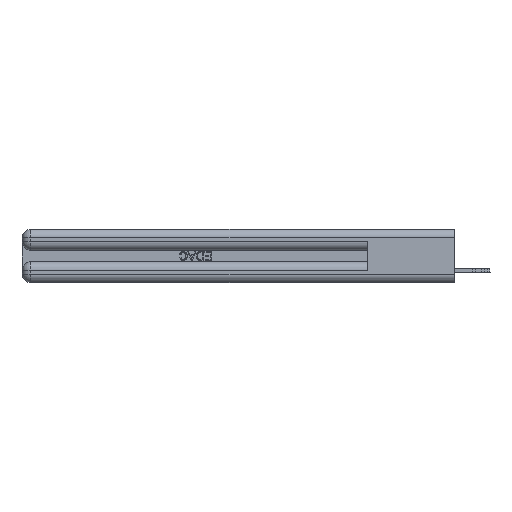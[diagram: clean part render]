
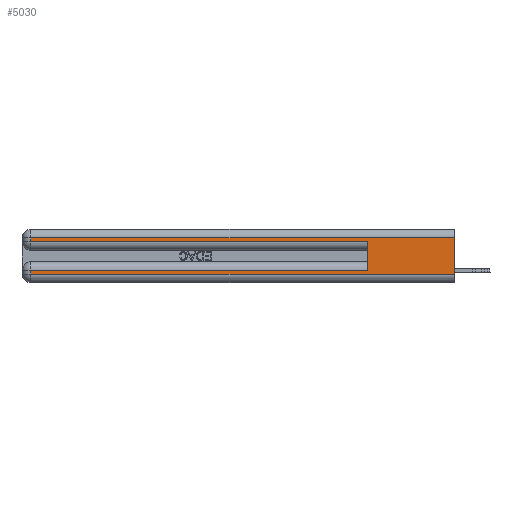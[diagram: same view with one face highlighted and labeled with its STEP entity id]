
A CAD part, left-side view. The second image highlights one B-rep face of the part: STEP entity #5030.
In plain terms, the highlighted planar face has unit normal (-1, 0, 0).
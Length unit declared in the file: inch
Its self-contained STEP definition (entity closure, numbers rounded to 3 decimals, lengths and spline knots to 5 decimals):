
#437 = CARTESIAN_POINT ( 'NONE',  ( 0., 2.94, 0.37 ) ) ;
#770 = DIRECTION ( 'NONE',  ( 1., 0., 0. ) ) ;
#1488 = EDGE_CURVE ( 'NONE', #3719, #33987, #32286, .T. ) ;
#1748 = EDGE_CURVE ( 'NONE', #42653, #26759, #40231, .T. ) ;
#3719 = VERTEX_POINT ( 'NONE', #22581 ) ;
#4705 = VERTEX_POINT ( 'NONE', #6514 ) ;
#5030 = ADVANCED_FACE ( 'NONE', ( #17092 ), #41225, .F. ) ;
#6514 = CARTESIAN_POINT ( 'NONE',  ( 0., 2.94, 0.31 ) ) ;
#7011 = EDGE_CURVE ( 'NONE', #24779, #18152, #34283, .T. ) ;
#9468 = VECTOR ( 'NONE', #13806, 39.37008 ) ;
#11278 = EDGE_CURVE ( 'NONE', #24779, #33987, #25274, .T. ) ;
#11892 = CARTESIAN_POINT ( 'NONE',  ( 0., 2.94, 0.06 ) ) ;
#11975 = DIRECTION ( 'NONE',  ( 0., 1., 0. ) ) ;
#12269 = VERTEX_POINT ( 'NONE', #37901 ) ;
#13163 = ORIENTED_EDGE ( 'NONE', *, *, #1748, .T. ) ;
#13584 = EDGE_CURVE ( 'NONE', #12269, #4705, #14735, .T. ) ;
#13806 = DIRECTION ( 'NONE',  ( 0., -1., 0. ) ) ;
#14131 = CARTESIAN_POINT ( 'NONE',  ( 0., 0.6, 0.285 ) ) ;
#14662 = ORIENTED_EDGE ( 'NONE', *, *, #11278, .F. ) ;
#14735 = LINE ( 'NONE', #26303, #24962 ) ;
#14923 = VECTOR ( 'NONE', #26394, 39.37008 ) ;
#15210 = ORIENTED_EDGE ( 'NONE', *, *, #1488, .T. ) ;
#15259 = AXIS2_PLACEMENT_3D ( 'NONE', #40905, #770, #33738 ) ;
#16176 = ORIENTED_EDGE ( 'NONE', *, *, #39527, .T. ) ;
#16331 = CARTESIAN_POINT ( 'NONE',  ( 0., 0., 0.06 ) ) ;
#17092 = FACE_OUTER_BOUND ( 'NONE', #43045, .T. ) ;
#18152 = VERTEX_POINT ( 'NONE', #25336 ) ;
#18877 = DIRECTION ( 'NONE',  ( 0., 0., 1. ) ) ;
#20898 = VECTOR ( 'NONE', #37984, 39.37008 ) ;
#21423 = DIRECTION ( 'NONE',  ( 0., 0., -1. ) ) ;
#22000 = DIRECTION ( 'NONE',  ( 0., 0., -1. ) ) ;
#22581 = CARTESIAN_POINT ( 'NONE',  ( 0., 2.94, 0.285 ) ) ;
#24779 = VERTEX_POINT ( 'NONE', #44823 ) ;
#24962 = VECTOR ( 'NONE', #11975, 39.37008 ) ;
#25274 = LINE ( 'NONE', #37369, #44666 ) ;
#25336 = CARTESIAN_POINT ( 'NONE',  ( 0., 2.94, 0.085 ) ) ;
#25928 = CARTESIAN_POINT ( 'NONE',  ( 0., 0., 0.085 ) ) ;
#26303 = CARTESIAN_POINT ( 'NONE',  ( 0., 0., 0.31 ) ) ;
#26394 = DIRECTION ( 'NONE',  ( 0., 1., 0. ) ) ;
#26427 = CARTESIAN_POINT ( 'NONE',  ( 0., 2.94, 0.37 ) ) ;
#26759 = VERTEX_POINT ( 'NONE', #33015 ) ;
#29350 = EDGE_CURVE ( 'NONE', #12269, #26759, #38855, .T. ) ;
#31267 = LINE ( 'NONE', #437, #42089 ) ;
#31501 = VECTOR ( 'NONE', #21423, 39.37008 ) ;
#31648 = EDGE_CURVE ( 'NONE', #4705, #3719, #31267, .T. ) ;
#32286 = LINE ( 'NONE', #46754, #9468 ) ;
#32737 = ORIENTED_EDGE ( 'NONE', *, *, #13584, .T. ) ;
#33015 = CARTESIAN_POINT ( 'NONE',  ( 0., 0., 0.06 ) ) ;
#33738 = DIRECTION ( 'NONE',  ( 0., 0., -1. ) ) ;
#33987 = VERTEX_POINT ( 'NONE', #14131 ) ;
#34283 = LINE ( 'NONE', #25928, #14923 ) ;
#36133 = ORIENTED_EDGE ( 'NONE', *, *, #7011, .T. ) ;
#37369 = CARTESIAN_POINT ( 'NONE',  ( 0., 0.6, 0.145 ) ) ;
#37901 = CARTESIAN_POINT ( 'NONE',  ( 0., 0., 0.31 ) ) ;
#37984 = DIRECTION ( 'NONE',  ( 0., -1., 0. ) ) ;
#38855 = LINE ( 'NONE', #43030, #31501 ) ;
#39137 = ORIENTED_EDGE ( 'NONE', *, *, #29350, .F. ) ;
#39527 = EDGE_CURVE ( 'NONE', #18152, #42653, #40462, .T. ) ;
#40231 = LINE ( 'NONE', #16331, #20898 ) ;
#40462 = LINE ( 'NONE', #26427, #43891 ) ;
#40905 = CARTESIAN_POINT ( 'NONE',  ( 0., 0., 0.37 ) ) ;
#41225 = PLANE ( 'NONE',  #15259 ) ;
#42089 = VECTOR ( 'NONE', #22000, 39.37008 ) ;
#42653 = VERTEX_POINT ( 'NONE', #11892 ) ;
#43030 = CARTESIAN_POINT ( 'NONE',  ( 0., 0., 0.37 ) ) ;
#43045 = EDGE_LOOP ( 'NONE', ( #39137, #32737, #46234, #15210, #14662, #36133, #16176, #13163 ) ) ;
#43891 = VECTOR ( 'NONE', #45050, 39.37008 ) ;
#44666 = VECTOR ( 'NONE', #18877, 39.37008 ) ;
#44823 = CARTESIAN_POINT ( 'NONE',  ( 0., 0.6, 0.085 ) ) ;
#45050 = DIRECTION ( 'NONE',  ( 0., 0., -1. ) ) ;
#46234 = ORIENTED_EDGE ( 'NONE', *, *, #31648, .T. ) ;
#46754 = CARTESIAN_POINT ( 'NONE',  ( 0., 0., 0.285 ) ) ;
